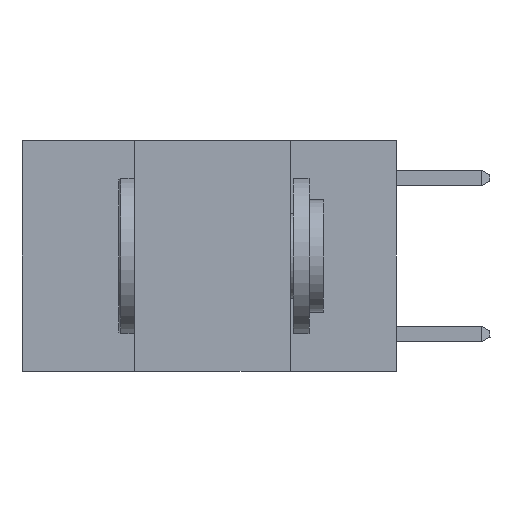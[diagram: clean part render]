
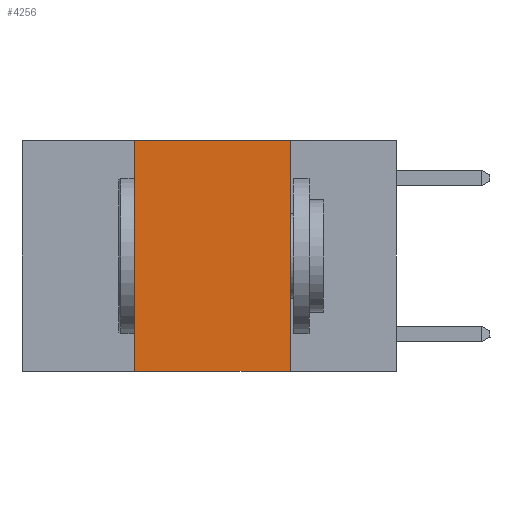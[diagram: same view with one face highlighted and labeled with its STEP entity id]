
A CAD part, left-side view. The second image highlights one B-rep face of the part: STEP entity #4256.
In plain terms, the highlighted planar face has unit normal (-1, 0, 0).
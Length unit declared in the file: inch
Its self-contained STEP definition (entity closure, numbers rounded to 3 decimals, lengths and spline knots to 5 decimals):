
#144 = PLANE ( 'NONE',  #10363 ) ;
#611 = CARTESIAN_POINT ( 'NONE',  ( 0., 0.6, -0.37 ) ) ;
#740 = ORIENTED_EDGE ( 'NONE', *, *, #7054, .F. ) ;
#753 = ORIENTED_EDGE ( 'NONE', *, *, #810, .F. ) ;
#810 = EDGE_CURVE ( 'NONE', #19400, #9070, #14826, .T. ) ;
#861 = ORIENTED_EDGE ( 'NONE', *, *, #7481, .F. ) ;
#877 = ORIENTED_EDGE ( 'NONE', *, *, #17732, .T. ) ;
#1883 = DIRECTION ( 'NONE',  ( 1., 0., 0. ) ) ;
#2392 = CARTESIAN_POINT ( 'NONE',  ( 0., 0.17, 0. ) ) ;
#2949 = CARTESIAN_POINT ( 'NONE',  ( 0., 0.6, 0. ) ) ;
#3024 = VECTOR ( 'NONE', #5427, 39.37008 ) ;
#3110 = LINE ( 'NONE', #16770, #3024 ) ;
#4256 = ADVANCED_FACE ( 'NONE', ( #18735 ), #144, .F. ) ;
#4600 = CARTESIAN_POINT ( 'NONE',  ( 0., 0.42, 0. ) ) ;
#5427 = DIRECTION ( 'NONE',  ( 0., 0., 1. ) ) ;
#5992 = VECTOR ( 'NONE', #18366, 39.37008 ) ;
#6071 = LINE ( 'NONE', #15271, #5992 ) ;
#6568 = CARTESIAN_POINT ( 'NONE',  ( 0., 0.42, -0.37 ) ) ;
#7054 = EDGE_CURVE ( 'NONE', #9070, #11911, #6071, .T. ) ;
#7481 = EDGE_CURVE ( 'NONE', #9347, #19400, #3110, .T. ) ;
#9070 = VERTEX_POINT ( 'NONE', #2392 ) ;
#9347 = VERTEX_POINT ( 'NONE', #6568 ) ;
#10363 = AXIS2_PLACEMENT_3D ( 'NONE', #12068, #1883, #13628 ) ;
#11640 = CARTESIAN_POINT ( 'NONE',  ( 0., 0.17, -0.37 ) ) ;
#11911 = VERTEX_POINT ( 'NONE', #11640 ) ;
#12068 = CARTESIAN_POINT ( 'NONE',  ( 0., 0.6, 0. ) ) ;
#12208 = LINE ( 'NONE', #611, #12679 ) ;
#12679 = VECTOR ( 'NONE', #13497, 39.37008 ) ;
#13497 = DIRECTION ( 'NONE',  ( 0., -1., 0. ) ) ;
#13628 = DIRECTION ( 'NONE',  ( 0., 0., -1. ) ) ;
#14379 = VECTOR ( 'NONE', #16123, 39.37008 ) ;
#14826 = LINE ( 'NONE', #2949, #14379 ) ;
#15271 = CARTESIAN_POINT ( 'NONE',  ( 0., 0.17, 0. ) ) ;
#16123 = DIRECTION ( 'NONE',  ( 0., -1., 0. ) ) ;
#16770 = CARTESIAN_POINT ( 'NONE',  ( 0., 0.42, 0. ) ) ;
#17732 = EDGE_CURVE ( 'NONE', #9347, #11911, #12208, .T. ) ;
#18185 = EDGE_LOOP ( 'NONE', ( #740, #753, #861, #877 ) ) ;
#18366 = DIRECTION ( 'NONE',  ( 0., 0., -1. ) ) ;
#18735 = FACE_OUTER_BOUND ( 'NONE', #18185, .T. ) ;
#19400 = VERTEX_POINT ( 'NONE', #4600 ) ;
